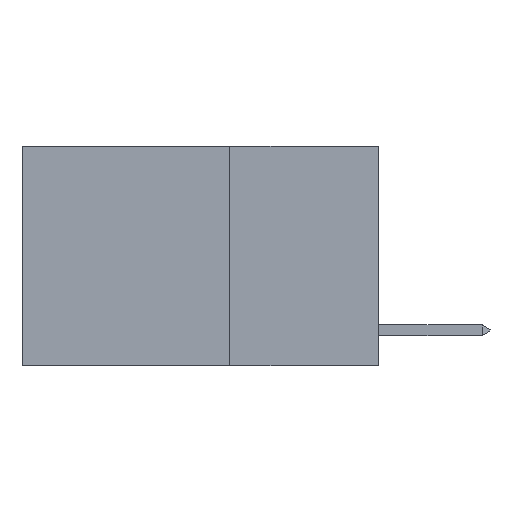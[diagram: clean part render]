
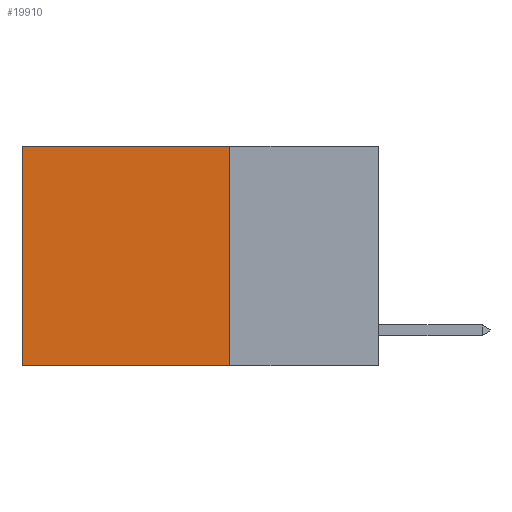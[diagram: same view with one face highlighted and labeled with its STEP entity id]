
A CAD part, left-side view. The second image highlights one B-rep face of the part: STEP entity #19910.
In plain terms, the highlighted planar face has unit normal (-1, 0, 0).
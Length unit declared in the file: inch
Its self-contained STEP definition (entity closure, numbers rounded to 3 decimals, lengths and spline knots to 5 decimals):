
#469 = FACE_OUTER_BOUND ( 'NONE', #22245, .T. ) ;
#528 = VECTOR ( 'NONE', #16433, 39.37008 ) ;
#662 = VERTEX_POINT ( 'NONE', #24372 ) ;
#2865 = CARTESIAN_POINT ( 'NONE',  ( 0.2625, 0.25, -0.37 ) ) ;
#3116 = LINE ( 'NONE', #16019, #16496 ) ;
#3683 = LINE ( 'NONE', #14153, #528 ) ;
#7087 = EDGE_CURVE ( 'NONE', #27116, #662, #3116, .T. ) ;
#7284 = CARTESIAN_POINT ( 'NONE',  ( 0.2625, 0.25, -0.37 ) ) ;
#10274 = CARTESIAN_POINT ( 'NONE',  ( 0.2625, 0.6, -0.37 ) ) ;
#11238 = VECTOR ( 'NONE', #17332, 39.37008 ) ;
#11486 = CARTESIAN_POINT ( 'NONE',  ( 0.2625, 0.25, 0. ) ) ;
#11952 = VECTOR ( 'NONE', #13885, 39.37008 ) ;
#12873 = CARTESIAN_POINT ( 'NONE',  ( 0.2625, 0.6, 0. ) ) ;
#13178 = ORIENTED_EDGE ( 'NONE', *, *, #24250, .F. ) ;
#13885 = DIRECTION ( 'NONE',  ( 0., 1., 0. ) ) ;
#14055 = ORIENTED_EDGE ( 'NONE', *, *, #7087, .T. ) ;
#14153 = CARTESIAN_POINT ( 'NONE',  ( 0.2625, 0.25, 0. ) ) ;
#14784 = LINE ( 'NONE', #12873, #11238 ) ;
#14860 = AXIS2_PLACEMENT_3D ( 'NONE', #11486, #18300, #25071 ) ;
#15304 = EDGE_CURVE ( 'NONE', #662, #22578, #14784, .T. ) ;
#16019 = CARTESIAN_POINT ( 'NONE',  ( 0.2625, 0.25, 0. ) ) ;
#16198 = DIRECTION ( 'NONE',  ( 0., 1., 0. ) ) ;
#16433 = DIRECTION ( 'NONE',  ( 0., 0., -1. ) ) ;
#16496 = VECTOR ( 'NONE', #16198, 39.37008 ) ;
#17332 = DIRECTION ( 'NONE',  ( 0., 0., -1. ) ) ;
#18300 = DIRECTION ( 'NONE',  ( 1., 0., 0. ) ) ;
#18627 = CARTESIAN_POINT ( 'NONE',  ( 0.2625, 0.25, 0. ) ) ;
#19290 = VERTEX_POINT ( 'NONE', #2865 ) ;
#19334 = ORIENTED_EDGE ( 'NONE', *, *, #15304, .T. ) ;
#19910 = ADVANCED_FACE ( 'NONE', ( #469 ), #24973, .F. ) ;
#20483 = ORIENTED_EDGE ( 'NONE', *, *, #26529, .F. ) ;
#22245 = EDGE_LOOP ( 'NONE', ( #19334, #20483, #13178, #14055 ) ) ;
#22578 = VERTEX_POINT ( 'NONE', #10274 ) ;
#22887 = LINE ( 'NONE', #7284, #11952 ) ;
#24250 = EDGE_CURVE ( 'NONE', #27116, #19290, #3683, .T. ) ;
#24372 = CARTESIAN_POINT ( 'NONE',  ( 0.2625, 0.6, 0. ) ) ;
#24973 = PLANE ( 'NONE',  #14860 ) ;
#25071 = DIRECTION ( 'NONE',  ( 0., 0., -1. ) ) ;
#26529 = EDGE_CURVE ( 'NONE', #19290, #22578, #22887, .T. ) ;
#27116 = VERTEX_POINT ( 'NONE', #18627 ) ;
